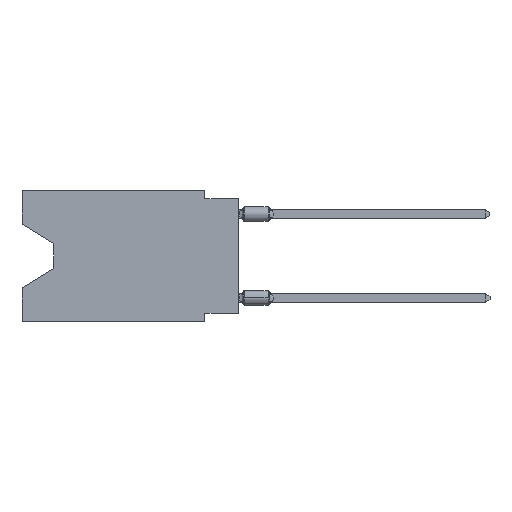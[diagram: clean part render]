
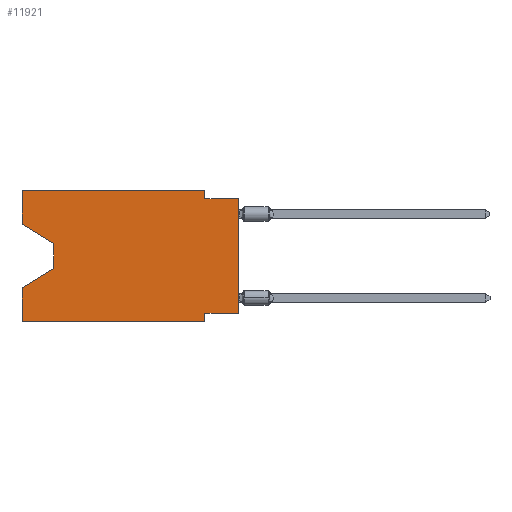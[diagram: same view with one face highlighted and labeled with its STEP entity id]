
A CAD part, left-side view. The second image highlights one B-rep face of the part: STEP entity #11921.
In plain terms, the highlighted planar face has unit normal (-1, 0, 0).
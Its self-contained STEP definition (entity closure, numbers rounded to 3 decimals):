
#7 = EDGE_LOOP ( 'NONE', ( #17145, #9794, #10935, #5977, #1454, #5926, #8706, #1732, #16863, #17496, #18673, #10416 ) ) ;
#180 = VECTOR ( 'NONE', #15483, 1000. ) ;
#313 = VECTOR ( 'NONE', #5217, 1000. ) ;
#457 = DIRECTION ( 'NONE',  ( 0., 0., 1. ) ) ;
#531 = CARTESIAN_POINT ( 'NONE',  ( 0., 16.383, -2.546 ) ) ;
#821 = VERTEX_POINT ( 'NONE', #8325 ) ;
#1003 = VECTOR ( 'NONE', #5406, 1000. ) ;
#1454 = ORIENTED_EDGE ( 'NONE', *, *, #18957, .T. ) ;
#1514 = CARTESIAN_POINT ( 'NONE',  ( 0., 0., -0.635 ) ) ;
#1577 = EDGE_CURVE ( 'NONE', #5779, #7453, #19045, .T. ) ;
#1579 = CARTESIAN_POINT ( 'NONE',  ( 0., 2.54, -9.271 ) ) ;
#1652 = CARTESIAN_POINT ( 'NONE',  ( 0., 0., -0.635 ) ) ;
#1704 = CARTESIAN_POINT ( 'NONE',  ( 0., 16.383, 0. ) ) ;
#1732 = ORIENTED_EDGE ( 'NONE', *, *, #4917, .T. ) ;
#1853 = CARTESIAN_POINT ( 'NONE',  ( 0., 16.383, -9.906 ) ) ;
#2360 = CARTESIAN_POINT ( 'NONE',  ( 0., 2.54, -9.906 ) ) ;
#2673 = VECTOR ( 'NONE', #19665, 1000. ) ;
#2729 = VECTOR ( 'NONE', #457, 1000. ) ;
#3023 = LINE ( 'NONE', #5770, #9693 ) ;
#3176 = LINE ( 'NONE', #1652, #9762 ) ;
#3613 = LINE ( 'NONE', #17255, #2729 ) ;
#4190 = DIRECTION ( 'NONE',  ( 1., 0., 0. ) ) ;
#4388 = FACE_OUTER_BOUND ( 'NONE', #7, .T. ) ;
#4431 = LINE ( 'NONE', #10568, #19945 ) ;
#4534 = CARTESIAN_POINT ( 'NONE',  ( 0., 2.54, -9.906 ) ) ;
#4917 = EDGE_CURVE ( 'NONE', #821, #14487, #3613, .T. ) ;
#5164 = EDGE_CURVE ( 'NONE', #6420, #14174, #5237, .T. ) ;
#5217 = DIRECTION ( 'NONE',  ( 0., -0.855, -0.519 ) ) ;
#5237 = LINE ( 'NONE', #11370, #8873 ) ;
#5406 = DIRECTION ( 'NONE',  ( 0., 0., 1. ) ) ;
#5429 = VERTEX_POINT ( 'NONE', #18225 ) ;
#5508 = VECTOR ( 'NONE', #10918, 1000. ) ;
#5770 = CARTESIAN_POINT ( 'NONE',  ( 0., 2.54, 0. ) ) ;
#5779 = VERTEX_POINT ( 'NONE', #12232 ) ;
#5849 = CARTESIAN_POINT ( 'NONE',  ( 0., 13.97, -4.013 ) ) ;
#5926 = ORIENTED_EDGE ( 'NONE', *, *, #6961, .F. ) ;
#5977 = ORIENTED_EDGE ( 'NONE', *, *, #9839, .F. ) ;
#6272 = LINE ( 'NONE', #1704, #7714 ) ;
#6420 = VERTEX_POINT ( 'NONE', #17770 ) ;
#6908 = LINE ( 'NONE', #7013, #1003 ) ;
#6961 = EDGE_CURVE ( 'NONE', #11164, #16639, #9829, .T. ) ;
#7013 = CARTESIAN_POINT ( 'NONE',  ( 0., 16.383, 0. ) ) ;
#7453 = VERTEX_POINT ( 'NONE', #8604 ) ;
#7511 = PLANE ( 'NONE',  #11198 ) ;
#7714 = VECTOR ( 'NONE', #9399, 1000. ) ;
#8325 = CARTESIAN_POINT ( 'NONE',  ( 0., 0., -9.271 ) ) ;
#8604 = CARTESIAN_POINT ( 'NONE',  ( 0., 13.97, -4.013 ) ) ;
#8706 = ORIENTED_EDGE ( 'NONE', *, *, #14565, .F. ) ;
#8873 = VECTOR ( 'NONE', #17542, 1000. ) ;
#9186 = DIRECTION ( 'NONE',  ( 0., 0., -1. ) ) ;
#9328 = LINE ( 'NONE', #1853, #180 ) ;
#9399 = DIRECTION ( 'NONE',  ( 0., -1., 0. ) ) ;
#9674 = CARTESIAN_POINT ( 'NONE',  ( 0., 16.383, 0. ) ) ;
#9693 = VECTOR ( 'NONE', #9186, 1000. ) ;
#9696 = CARTESIAN_POINT ( 'NONE',  ( 0., 16.383, -9.906 ) ) ;
#9762 = VECTOR ( 'NONE', #13982, 1000. ) ;
#9794 = ORIENTED_EDGE ( 'NONE', *, *, #16480, .T. ) ;
#9829 = LINE ( 'NONE', #2360, #18184 ) ;
#9839 = EDGE_CURVE ( 'NONE', #10767, #14174, #4431, .T. ) ;
#10416 = ORIENTED_EDGE ( 'NONE', *, *, #12984, .F. ) ;
#10568 = CARTESIAN_POINT ( 'NONE',  ( 0., 16.383, 0. ) ) ;
#10628 = DIRECTION ( 'NONE',  ( 0., 0., -1. ) ) ;
#10671 = DIRECTION ( 'NONE',  ( 0., 0., 1. ) ) ;
#10702 = EDGE_CURVE ( 'NONE', #11217, #18015, #6272, .T. ) ;
#10767 = VERTEX_POINT ( 'NONE', #9696 ) ;
#10918 = DIRECTION ( 'NONE',  ( 0., 1., 0. ) ) ;
#10935 = ORIENTED_EDGE ( 'NONE', *, *, #5164, .T. ) ;
#11164 = VERTEX_POINT ( 'NONE', #1579 ) ;
#11198 = AXIS2_PLACEMENT_3D ( 'NONE', #18112, #4190, #10628 ) ;
#11217 = VERTEX_POINT ( 'NONE', #9674 ) ;
#11370 = CARTESIAN_POINT ( 'NONE',  ( 0., 13.97, -5.893 ) ) ;
#11921 = ADVANCED_FACE ( 'NONE', ( #4388 ), #7511, .F. ) ;
#12232 = CARTESIAN_POINT ( 'NONE',  ( 0., 16.383, -2.546 ) ) ;
#12434 = LINE ( 'NONE', #15463, #5508 ) ;
#12984 = EDGE_CURVE ( 'NONE', #5779, #11217, #6908, .T. ) ;
#13728 = CARTESIAN_POINT ( 'NONE',  ( 0., 2.54, 0. ) ) ;
#13811 = LINE ( 'NONE', #5849, #2673 ) ;
#13982 = DIRECTION ( 'NONE',  ( 0., -1., 0. ) ) ;
#14174 = VERTEX_POINT ( 'NONE', #16000 ) ;
#14487 = VERTEX_POINT ( 'NONE', #1514 ) ;
#14565 = EDGE_CURVE ( 'NONE', #821, #11164, #12434, .T. ) ;
#14758 = EDGE_CURVE ( 'NONE', #18015, #5429, #3023, .T. ) ;
#15463 = CARTESIAN_POINT ( 'NONE',  ( 0., 0., -9.271 ) ) ;
#15483 = DIRECTION ( 'NONE',  ( 0., -1., 0. ) ) ;
#15795 = DIRECTION ( 'NONE',  ( 0., 0., -1. ) ) ;
#15804 = EDGE_CURVE ( 'NONE', #5429, #14487, #3176, .T. ) ;
#16000 = CARTESIAN_POINT ( 'NONE',  ( 0., 16.383, -7.36 ) ) ;
#16480 = EDGE_CURVE ( 'NONE', #7453, #6420, #13811, .T. ) ;
#16639 = VERTEX_POINT ( 'NONE', #4534 ) ;
#16863 = ORIENTED_EDGE ( 'NONE', *, *, #15804, .F. ) ;
#17145 = ORIENTED_EDGE ( 'NONE', *, *, #1577, .T. ) ;
#17255 = CARTESIAN_POINT ( 'NONE',  ( 0., 0., 0. ) ) ;
#17496 = ORIENTED_EDGE ( 'NONE', *, *, #14758, .F. ) ;
#17542 = DIRECTION ( 'NONE',  ( 0., 0.855, -0.519 ) ) ;
#17770 = CARTESIAN_POINT ( 'NONE',  ( 0., 13.97, -5.893 ) ) ;
#18015 = VERTEX_POINT ( 'NONE', #13728 ) ;
#18112 = CARTESIAN_POINT ( 'NONE',  ( 0., 16.383, 0. ) ) ;
#18184 = VECTOR ( 'NONE', #15795, 1000. ) ;
#18225 = CARTESIAN_POINT ( 'NONE',  ( 0., 2.54, -0.635 ) ) ;
#18673 = ORIENTED_EDGE ( 'NONE', *, *, #10702, .F. ) ;
#18957 = EDGE_CURVE ( 'NONE', #10767, #16639, #9328, .T. ) ;
#19045 = LINE ( 'NONE', #531, #313 ) ;
#19665 = DIRECTION ( 'NONE',  ( 0., 0., -1. ) ) ;
#19945 = VECTOR ( 'NONE', #10671, 1000. ) ;
